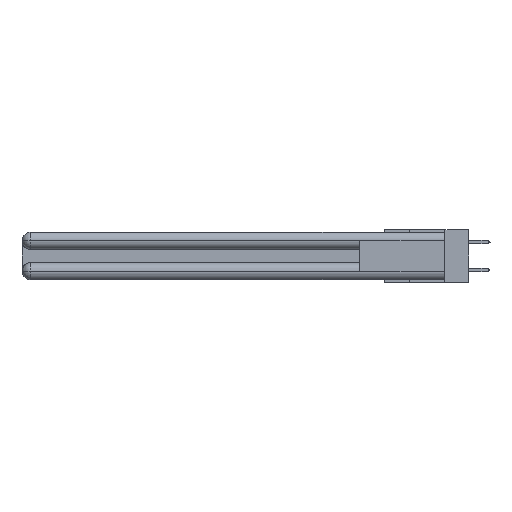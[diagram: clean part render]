
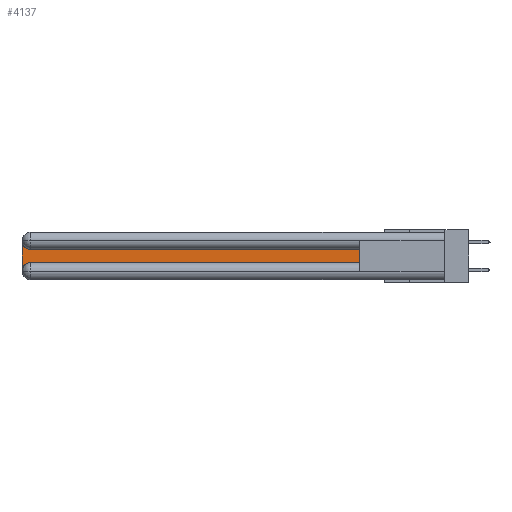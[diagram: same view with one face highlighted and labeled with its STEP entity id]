
A CAD part, left-side view. The second image highlights one B-rep face of the part: STEP entity #4137.
In plain terms, the highlighted planar face has unit normal (-1, 0, 0).
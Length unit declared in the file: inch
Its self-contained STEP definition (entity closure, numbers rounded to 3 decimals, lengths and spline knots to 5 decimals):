
#1383 = VERTEX_POINT ( 'NONE', #21704 ) ;
#1534 = CARTESIAN_POINT ( 'NONE',  ( 0.075, 2.94, -0.2775 ) ) ;
#2198 = CIRCLE ( 'NONE', #10999, 0.06 ) ;
#2403 = LINE ( 'NONE', #24531, #26500 ) ;
#2507 = CARTESIAN_POINT ( 'NONE',  ( 0.075, 0.6, -0.2175 ) ) ;
#2965 = FACE_OUTER_BOUND ( 'NONE', #17552, .T. ) ;
#3525 = VERTEX_POINT ( 'NONE', #13600 ) ;
#3888 = DIRECTION ( 'NONE',  ( 0., 1., 0. ) ) ;
#4137 = ADVANCED_FACE ( 'NONE', ( #2965 ), #18134, .F. ) ;
#5444 = ORIENTED_EDGE ( 'NONE', *, *, #6930, .T. ) ;
#6930 = EDGE_CURVE ( 'NONE', #15373, #26401, #2403, .T. ) ;
#8361 = VERTEX_POINT ( 'NONE', #11546 ) ;
#8436 = DIRECTION ( 'NONE',  ( 1., 0., 0. ) ) ;
#8789 = CIRCLE ( 'NONE', #10424, 0.06 ) ;
#9250 = AXIS2_PLACEMENT_3D ( 'NONE', #22403, #8436, #29947 ) ;
#9892 = DIRECTION ( 'NONE',  ( 0., 0., -1. ) ) ;
#10424 = AXIS2_PLACEMENT_3D ( 'NONE', #1534, #26892, #27281 ) ;
#10999 = AXIS2_PLACEMENT_3D ( 'NONE', #15267, #26995, #22064 ) ;
#11546 = CARTESIAN_POINT ( 'NONE',  ( 0.075, 3., -0.2775 ) ) ;
#11738 = DIRECTION ( 'NONE',  ( 0., 0., 1. ) ) ;
#12460 = VECTOR ( 'NONE', #21676, 39.37008 ) ;
#13209 = LINE ( 'NONE', #23298, #12460 ) ;
#13600 = CARTESIAN_POINT ( 'NONE',  ( 0.075, 0.6, -0.2175 ) ) ;
#14669 = EDGE_CURVE ( 'NONE', #26401, #1383, #2198, .T. ) ;
#15267 = CARTESIAN_POINT ( 'NONE',  ( 0.075, 2.94, -0.0625 ) ) ;
#15274 = EDGE_CURVE ( 'NONE', #3525, #15373, #17486, .T. ) ;
#15373 = VERTEX_POINT ( 'NONE', #28487 ) ;
#16374 = VECTOR ( 'NONE', #11738, 39.37008 ) ;
#16578 = CARTESIAN_POINT ( 'NONE',  ( 0.075, 2.94, -0.1225 ) ) ;
#16640 = CARTESIAN_POINT ( 'NONE',  ( 0.075, 3., -0.2175 ) ) ;
#17486 = LINE ( 'NONE', #2507, #16374 ) ;
#17552 = EDGE_LOOP ( 'NONE', ( #5444, #23584, #20867, #26679, #24950, #18232 ) ) ;
#17620 = LINE ( 'NONE', #16640, #23421 ) ;
#18134 = PLANE ( 'NONE',  #9250 ) ;
#18232 = ORIENTED_EDGE ( 'NONE', *, *, #15274, .T. ) ;
#20867 = ORIENTED_EDGE ( 'NONE', *, *, #27001, .T. ) ;
#21676 = DIRECTION ( 'NONE',  ( 0., -1., 0. ) ) ;
#21704 = CARTESIAN_POINT ( 'NONE',  ( 0.075, 3., -0.0625 ) ) ;
#22064 = DIRECTION ( 'NONE',  ( 0., 0., -1. ) ) ;
#22096 = EDGE_CURVE ( 'NONE', #22777, #3525, #13209, .T. ) ;
#22403 = CARTESIAN_POINT ( 'NONE',  ( 0.075, 3., -0.1225 ) ) ;
#22777 = VERTEX_POINT ( 'NONE', #26842 ) ;
#23298 = CARTESIAN_POINT ( 'NONE',  ( 0.075, 0.6, -0.2175 ) ) ;
#23421 = VECTOR ( 'NONE', #9892, 39.37008 ) ;
#23584 = ORIENTED_EDGE ( 'NONE', *, *, #14669, .T. ) ;
#24531 = CARTESIAN_POINT ( 'NONE',  ( 0.075, 0.6, -0.1225 ) ) ;
#24950 = ORIENTED_EDGE ( 'NONE', *, *, #22096, .T. ) ;
#26401 = VERTEX_POINT ( 'NONE', #16578 ) ;
#26500 = VECTOR ( 'NONE', #3888, 39.37008 ) ;
#26679 = ORIENTED_EDGE ( 'NONE', *, *, #27715, .T. ) ;
#26842 = CARTESIAN_POINT ( 'NONE',  ( 0.075, 2.94, -0.2175 ) ) ;
#26892 = DIRECTION ( 'NONE',  ( 1., 0., 0. ) ) ;
#26995 = DIRECTION ( 'NONE',  ( 1., 0., 0. ) ) ;
#27001 = EDGE_CURVE ( 'NONE', #1383, #8361, #17620, .T. ) ;
#27281 = DIRECTION ( 'NONE',  ( 0., 0., -1. ) ) ;
#27715 = EDGE_CURVE ( 'NONE', #8361, #22777, #8789, .T. ) ;
#28487 = CARTESIAN_POINT ( 'NONE',  ( 0.075, 0.6, -0.1225 ) ) ;
#29947 = DIRECTION ( 'NONE',  ( 0., 0., -1. ) ) ;
